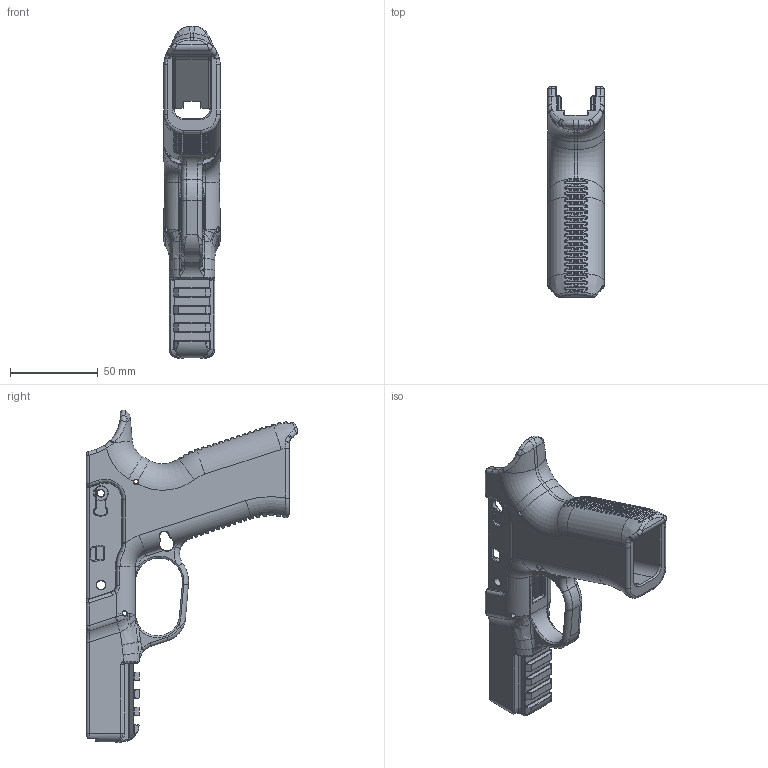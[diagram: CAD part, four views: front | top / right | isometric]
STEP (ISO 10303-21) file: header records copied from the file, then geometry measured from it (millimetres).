
FILE_DESCRIPTION(/* description */ (''),/* implementation_level */ '2;1');
FILE_NAME(/* name */ 'EAA SAR K2P.step',/* time_stamp */ '2019-11-17T17:53:54-05:00',/* author */ (''),/* organization */ (''),/* preprocessor_version */ 'ST-DEVELOPER v18',/* originating_system */ 'Autodesk Translation Framework v8.12.0.6',/* authorisation */ '');
FILE_SCHEMA (('AUTOMOTIVE_DESIGN { 1 0 10303 214 3 1 1 }'));
Products named in the file (1): EAA SAR K2P
Bounding box: 32 x 120.27 x 189.16 mm (x, y, z)
Volume: 119047.9 mm3; surface area: 52064.9 mm2
Topology: 1 solids, 1 shells, 1629 faces, 4016 edges, 2324 vertices
Faces by surface type: bspline 638, cylinder 516, plane 243, torus 154, sphere 44, cone 34
Full cylindrical faces by diameter (mm): 2.5 x5, 2.75 x1, 4 x1, 5 x2, 5.375 x1, 8 x1
Entity records: 67124 total; most frequent: CARTESIAN_POINT 31517, ORIENTED_EDGE 7948, DIRECTION 6844, EDGE_CURVE 3974, AXIS2_PLACEMENT_3D 2854, VERTEX_POINT 2325, EDGE_LOOP 1639, FACE_OUTER_BOUND 1629
